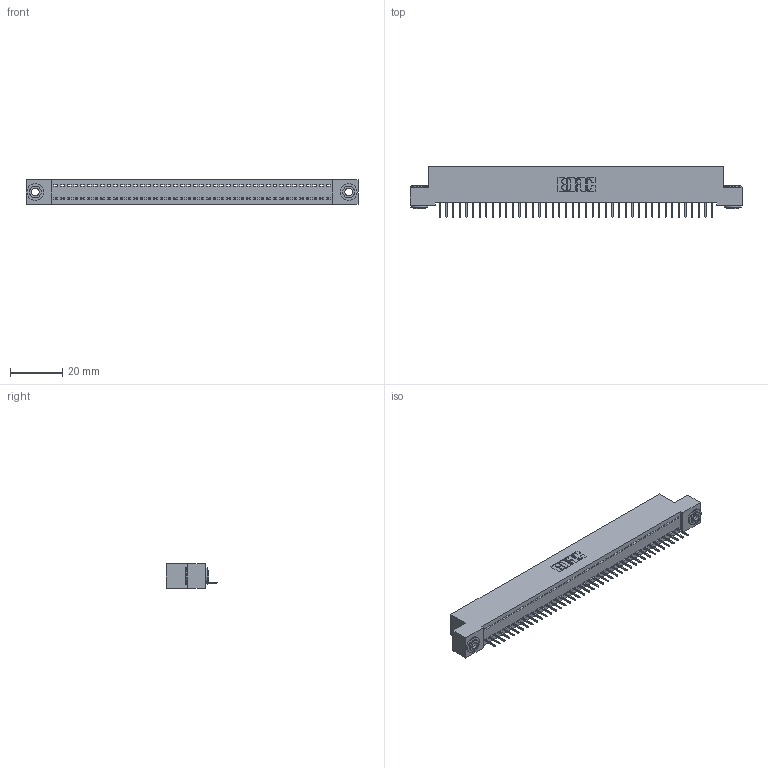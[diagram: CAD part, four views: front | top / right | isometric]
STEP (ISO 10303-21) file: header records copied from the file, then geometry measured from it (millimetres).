
FILE_DESCRIPTION (( 'STEP AP203' ), '1' );
FILE_NAME ('342-042-524-103.STEP', '2019-10-02T17:50:12', ( '' ), ( '' ), 'SwSTEP 2.0', 'SolidWorks 2016', '' );
FILE_SCHEMA (( 'CONFIG_CONTROL_DESIGN' ));
Length unit declared in the file: inch
Products named in the file (4): 342-250-002_345-250-002-102; 342-042-524-103; 342 Part_.156 TH; 345-292-001_345-293-124
Assembly tree (45 placements, depth 2):
  342-042-524-103
    342 Part_.156 TH
    345-292-001_345-293-124  x42
    342-250-002_345-250-002-102  x2
Bounding box: 127 x 19.69 x 9.4 mm (x, y, z)
Volume: 10992.3 mm3; surface area: 15852.5 mm2
Topology: 45 solids, 45 shells, 2752 faces, 7935 edges, 5118 vertices
Faces by surface type: plane 2092, cylinder 652, cone 8
Entity records: 26268 total; most frequent: CARTESIAN_POINT 4507, ORIENTED_EDGE 4478, DIRECTION 3837, EDGE_CURVE 2239, LINE 2091, VECTOR 2091, VERTEX_POINT 1486, AXIS2_PLACEMENT_3D 873
